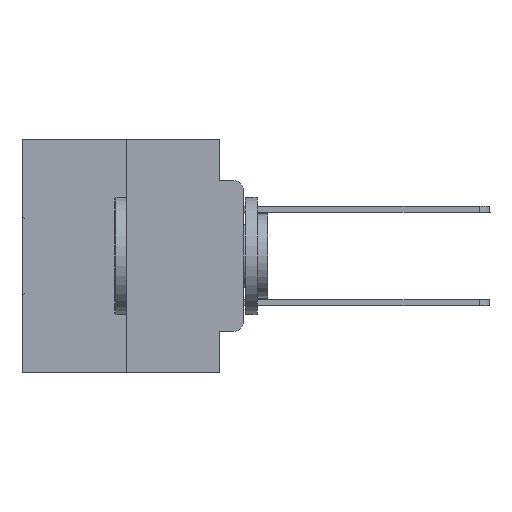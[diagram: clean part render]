
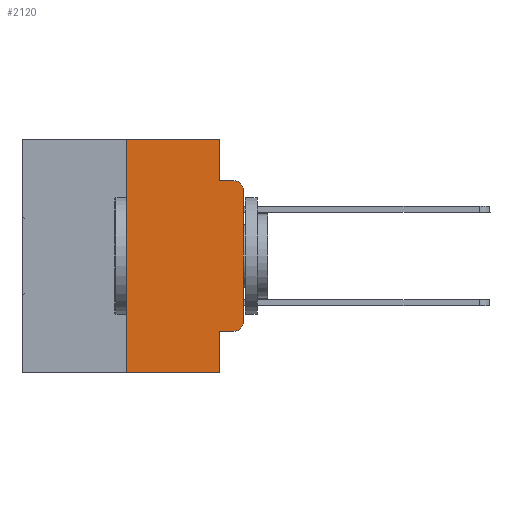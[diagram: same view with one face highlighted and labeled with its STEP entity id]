
A CAD part, left-side view. The second image highlights one B-rep face of the part: STEP entity #2120.
In plain terms, the highlighted planar face has unit normal (-1, 0, 0).
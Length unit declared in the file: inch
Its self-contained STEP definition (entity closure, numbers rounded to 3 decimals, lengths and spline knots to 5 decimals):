
#95 = LINE ( 'NONE', #4679, #4038 ) ;
#238 = ORIENTED_EDGE ( 'NONE', *, *, #26007, .F. ) ;
#972 = CARTESIAN_POINT ( 'NONE',  ( 0., 0.02, -0.0885 ) ) ;
#1521 = LINE ( 'NONE', #6590, #9007 ) ;
#2070 = DIRECTION ( 'NONE',  ( 0., 0., 1. ) ) ;
#2120 = ADVANCED_FACE ( 'NONE', ( #8516 ), #16314, .F. ) ;
#2428 = CARTESIAN_POINT ( 'NONE',  ( 0., 0.051, -0.0885 ) ) ;
#2732 = LINE ( 'NONE', #2428, #6021 ) ;
#3594 = DIRECTION ( 'NONE',  ( 0., 0., -1. ) ) ;
#3934 = VERTEX_POINT ( 'NONE', #25950 ) ;
#4038 = VECTOR ( 'NONE', #2070, 39.37008 ) ;
#4078 = EDGE_CURVE ( 'NONE', #28726, #29194, #31468, .T. ) ;
#4430 = CARTESIAN_POINT ( 'NONE',  ( 0., 0.051, 0. ) ) ;
#4679 = CARTESIAN_POINT ( 'NONE',  ( 0., 0., 0. ) ) ;
#5530 = VERTEX_POINT ( 'NONE', #15476 ) ;
#5550 = CARTESIAN_POINT ( 'NONE',  ( 0., 0.051, -0.0885 ) ) ;
#5751 = CARTESIAN_POINT ( 'NONE',  ( 0., 0.051, -0.4115 ) ) ;
#5810 = CARTESIAN_POINT ( 'NONE',  ( 0., 0.051, -0.4115 ) ) ;
#5845 = CARTESIAN_POINT ( 'NONE',  ( 0., 0.051, 0. ) ) ;
#6021 = VECTOR ( 'NONE', #19721, 39.37008 ) ;
#6322 = VECTOR ( 'NONE', #11489, 39.37008 ) ;
#6412 = CIRCLE ( 'NONE', #25713, 0.02 ) ;
#6590 = CARTESIAN_POINT ( 'NONE',  ( 0., 0.25, 0. ) ) ;
#6601 = ORIENTED_EDGE ( 'NONE', *, *, #17466, .T. ) ;
#7037 = ORIENTED_EDGE ( 'NONE', *, *, #27673, .F. ) ;
#8516 = FACE_OUTER_BOUND ( 'NONE', #15265, .T. ) ;
#8854 = VERTEX_POINT ( 'NONE', #28007 ) ;
#9007 = VECTOR ( 'NONE', #13801, 39.37008 ) ;
#9043 = AXIS2_PLACEMENT_3D ( 'NONE', #28730, #18448, #3594 ) ;
#9817 = EDGE_CURVE ( 'NONE', #28127, #8854, #23312, .T. ) ;
#9925 = EDGE_CURVE ( 'NONE', #26691, #25122, #2732, .T. ) ;
#10902 = DIRECTION ( 'NONE',  ( 0., -1., 0. ) ) ;
#11489 = DIRECTION ( 'NONE',  ( 0., -1., 0. ) ) ;
#12541 = EDGE_CURVE ( 'NONE', #25616, #26691, #24040, .T. ) ;
#13287 = AXIS2_PLACEMENT_3D ( 'NONE', #29324, #19210, #19852 ) ;
#13801 = DIRECTION ( 'NONE',  ( 0., 0., 1. ) ) ;
#14504 = VECTOR ( 'NONE', #21115, 39.37008 ) ;
#14838 = CARTESIAN_POINT ( 'NONE',  ( 0., 0.25, -0.5 ) ) ;
#15265 = EDGE_LOOP ( 'NONE', ( #23586, #25075, #21598, #22764, #7037, #238, #28167, #30609, #6601, #25283 ) ) ;
#15476 = CARTESIAN_POINT ( 'NONE',  ( 0., 0., -0.1085 ) ) ;
#16203 = LINE ( 'NONE', #16524, #6322 ) ;
#16314 = PLANE ( 'NONE',  #9043 ) ;
#16524 = CARTESIAN_POINT ( 'NONE',  ( 0., 0.473, 0. ) ) ;
#16947 = VECTOR ( 'NONE', #30305, 39.37008 ) ;
#17454 = EDGE_CURVE ( 'NONE', #22079, #8854, #30762, .T. ) ;
#17466 = EDGE_CURVE ( 'NONE', #28127, #28726, #28165, .T. ) ;
#18448 = DIRECTION ( 'NONE',  ( 1., 0., 0. ) ) ;
#19113 = DIRECTION ( 'NONE',  ( -1., 0., 0. ) ) ;
#19210 = DIRECTION ( 'NONE',  ( -1., 0., 0. ) ) ;
#19420 = EDGE_CURVE ( 'NONE', #29194, #5530, #95, .T. ) ;
#19721 = DIRECTION ( 'NONE',  ( 0., -1., 0. ) ) ;
#19852 = DIRECTION ( 'NONE',  ( 0., 0., -1. ) ) ;
#21115 = DIRECTION ( 'NONE',  ( 0., 0., -1. ) ) ;
#21290 = CARTESIAN_POINT ( 'NONE',  ( 0., 0.473, -0.5 ) ) ;
#21598 = ORIENTED_EDGE ( 'NONE', *, *, #9925, .F. ) ;
#22079 = VERTEX_POINT ( 'NONE', #14838 ) ;
#22149 = VECTOR ( 'NONE', #10902, 39.37008 ) ;
#22428 = CARTESIAN_POINT ( 'NONE',  ( 0., 0.02, -0.4115 ) ) ;
#22764 = ORIENTED_EDGE ( 'NONE', *, *, #12541, .F. ) ;
#23312 = LINE ( 'NONE', #5845, #16947 ) ;
#23586 = ORIENTED_EDGE ( 'NONE', *, *, #19420, .T. ) ;
#24040 = LINE ( 'NONE', #4430, #14504 ) ;
#24765 = VECTOR ( 'NONE', #25712, 39.37008 ) ;
#25075 = ORIENTED_EDGE ( 'NONE', *, *, #31185, .T. ) ;
#25122 = VERTEX_POINT ( 'NONE', #972 ) ;
#25283 = ORIENTED_EDGE ( 'NONE', *, *, #4078, .T. ) ;
#25616 = VERTEX_POINT ( 'NONE', #30948 ) ;
#25712 = DIRECTION ( 'NONE',  ( 0., -1., 0. ) ) ;
#25713 = AXIS2_PLACEMENT_3D ( 'NONE', #29570, #19113, #31689 ) ;
#25950 = CARTESIAN_POINT ( 'NONE',  ( 0., 0.25, 0. ) ) ;
#26007 = EDGE_CURVE ( 'NONE', #22079, #3934, #1521, .T. ) ;
#26691 = VERTEX_POINT ( 'NONE', #5550 ) ;
#27673 = EDGE_CURVE ( 'NONE', #3934, #25616, #16203, .T. ) ;
#27955 = CARTESIAN_POINT ( 'NONE',  ( 0., 0., -0.3915 ) ) ;
#28007 = CARTESIAN_POINT ( 'NONE',  ( 0., 0.051, -0.5 ) ) ;
#28127 = VERTEX_POINT ( 'NONE', #5751 ) ;
#28165 = LINE ( 'NONE', #5810, #24765 ) ;
#28167 = ORIENTED_EDGE ( 'NONE', *, *, #17454, .T. ) ;
#28726 = VERTEX_POINT ( 'NONE', #22428 ) ;
#28730 = CARTESIAN_POINT ( 'NONE',  ( 0., 0.473, 0. ) ) ;
#29194 = VERTEX_POINT ( 'NONE', #27955 ) ;
#29324 = CARTESIAN_POINT ( 'NONE',  ( 0., 0.02, -0.3915 ) ) ;
#29570 = CARTESIAN_POINT ( 'NONE',  ( 0., 0.02, -0.1085 ) ) ;
#30305 = DIRECTION ( 'NONE',  ( 0., 0., -1. ) ) ;
#30609 = ORIENTED_EDGE ( 'NONE', *, *, #9817, .F. ) ;
#30762 = LINE ( 'NONE', #21290, #22149 ) ;
#30948 = CARTESIAN_POINT ( 'NONE',  ( 0., 0.051, 0. ) ) ;
#31185 = EDGE_CURVE ( 'NONE', #5530, #25122, #6412, .T. ) ;
#31468 = CIRCLE ( 'NONE', #13287, 0.02 ) ;
#31689 = DIRECTION ( 'NONE',  ( 0., 0., -1. ) ) ;
